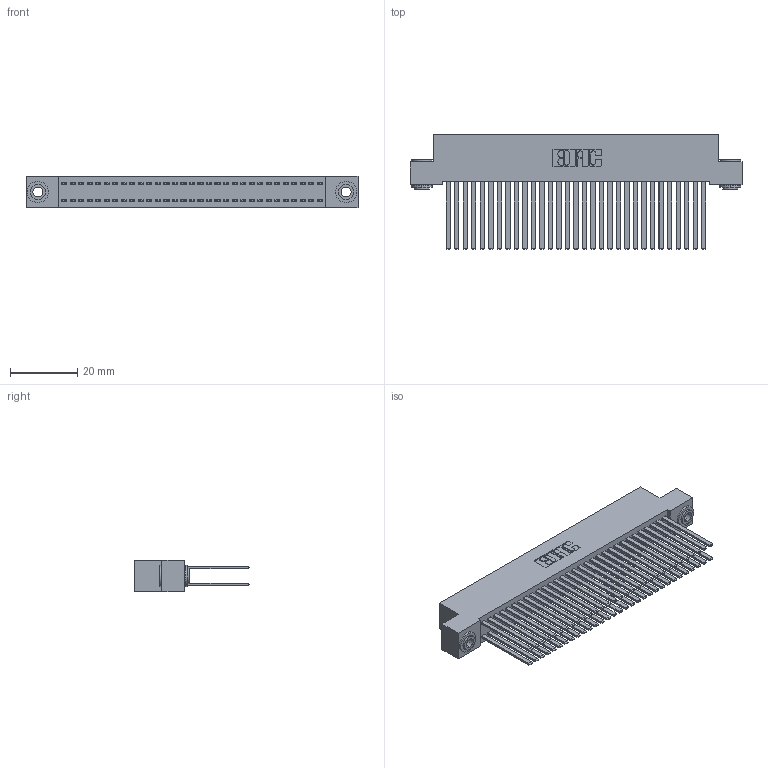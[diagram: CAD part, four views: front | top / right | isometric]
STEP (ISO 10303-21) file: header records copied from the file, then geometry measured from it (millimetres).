
FILE_DESCRIPTION (( 'STEP AP203' ), '1' );
FILE_NAME ('392-062-544-203.STEP', '2019-10-08T18:01:23', ( '' ), ( '' ), 'SwSTEP 2.0', 'SolidWorks 2016', '' );
FILE_SCHEMA (( 'CONFIG_CONTROL_DESIGN' ));
Length unit declared in the file: inch
Products named in the file (4): 392-062-544-203; 342 Part_.156 TH; 345-292-001_345-293-144; 342-250-002_345-250-002-102
Assembly tree (65 placements, depth 2):
  392-062-544-203
    342 Part_.156 TH
    345-292-001_345-293-144  x62
    342-250-002_345-250-002-102  x2
Bounding box: 99.06 x 34.3 x 9.4 mm (x, y, z)
Volume: 9740.4 mm3; surface area: 18204.9 mm2
Topology: 65 solids, 65 shells, 3000 faces, 8869 edges, 5826 vertices
Faces by surface type: plane 2060, cylinder 932, cone 8
Entity records: 21700 total; most frequent: CARTESIAN_POINT 3581, ORIENTED_EDGE 3510, DIRECTION 3109, EDGE_CURVE 1755, LINE 1607, VECTOR 1607, VERTEX_POINT 1166, AXIS2_PLACEMENT_3D 751
